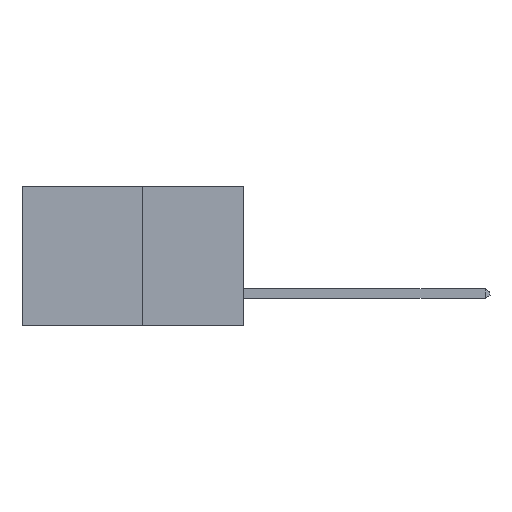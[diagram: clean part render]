
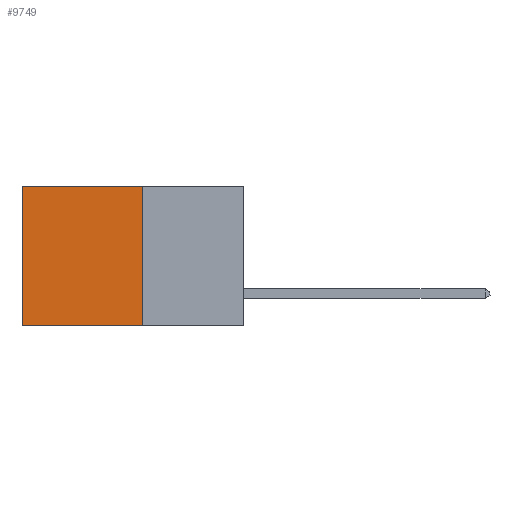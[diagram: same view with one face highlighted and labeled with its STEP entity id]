
A CAD part, left-side view. The second image highlights one B-rep face of the part: STEP entity #9749.
In plain terms, the highlighted planar face has unit normal (-1, 0, 0).
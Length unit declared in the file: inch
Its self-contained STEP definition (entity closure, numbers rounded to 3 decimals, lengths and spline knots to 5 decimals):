
#231 = CARTESIAN_POINT ( 'NONE',  ( 0.277, 0.59, -0.37 ) ) ;
#280 = EDGE_CURVE ( 'NONE', #4749, #3117, #490, .T. ) ;
#294 = ORIENTED_EDGE ( 'NONE', *, *, #6103, .F. ) ;
#366 = AXIS2_PLACEMENT_3D ( 'NONE', #7213, #4935, #9999 ) ;
#490 = LINE ( 'NONE', #6694, #4669 ) ;
#638 = VECTOR ( 'NONE', #7488, 39.37008 ) ;
#659 = EDGE_LOOP ( 'NONE', ( #2244, #294, #944, #1124 ) ) ;
#897 = FACE_OUTER_BOUND ( 'NONE', #659, .T. ) ;
#903 = CARTESIAN_POINT ( 'NONE',  ( 0.277, 0.59, -0.37 ) ) ;
#944 = ORIENTED_EDGE ( 'NONE', *, *, #9655, .F. ) ;
#1052 = VERTEX_POINT ( 'NONE', #7334 ) ;
#1124 = ORIENTED_EDGE ( 'NONE', *, *, #280, .T. ) ;
#1454 = LINE ( 'NONE', #2458, #9580 ) ;
#1643 = LINE ( 'NONE', #5140, #5436 ) ;
#2244 = ORIENTED_EDGE ( 'NONE', *, *, #9331, .T. ) ;
#2458 = CARTESIAN_POINT ( 'NONE',  ( 0.277, 0.27, -0.37 ) ) ;
#2934 = CARTESIAN_POINT ( 'NONE',  ( 0.277, 0.59, 0. ) ) ;
#3117 = VERTEX_POINT ( 'NONE', #2934 ) ;
#4669 = VECTOR ( 'NONE', #6974, 39.37008 ) ;
#4749 = VERTEX_POINT ( 'NONE', #7589 ) ;
#4935 = DIRECTION ( 'NONE',  ( 1., 0., 0. ) ) ;
#5140 = CARTESIAN_POINT ( 'NONE',  ( 0.277, 0.27, -0.37 ) ) ;
#5240 = DIRECTION ( 'NONE',  ( 0., 1., 0. ) ) ;
#5436 = VECTOR ( 'NONE', #5240, 39.37008 ) ;
#5691 = PLANE ( 'NONE',  #366 ) ;
#6103 = EDGE_CURVE ( 'NONE', #1052, #9825, #1643, .T. ) ;
#6694 = CARTESIAN_POINT ( 'NONE',  ( 0.277, 0.27, 0. ) ) ;
#6974 = DIRECTION ( 'NONE',  ( 0., 1., 0. ) ) ;
#7213 = CARTESIAN_POINT ( 'NONE',  ( 0.277, 0.27, -0.37 ) ) ;
#7293 = LINE ( 'NONE', #231, #638 ) ;
#7334 = CARTESIAN_POINT ( 'NONE',  ( 0.277, 0.27, -0.37 ) ) ;
#7488 = DIRECTION ( 'NONE',  ( 0., 0., -1. ) ) ;
#7589 = CARTESIAN_POINT ( 'NONE',  ( 0.277, 0.27, 0. ) ) ;
#7917 = DIRECTION ( 'NONE',  ( 0., 0., -1. ) ) ;
#9331 = EDGE_CURVE ( 'NONE', #3117, #9825, #7293, .T. ) ;
#9580 = VECTOR ( 'NONE', #7917, 39.37008 ) ;
#9655 = EDGE_CURVE ( 'NONE', #4749, #1052, #1454, .T. ) ;
#9749 = ADVANCED_FACE ( 'NONE', ( #897 ), #5691, .F. ) ;
#9825 = VERTEX_POINT ( 'NONE', #903 ) ;
#9999 = DIRECTION ( 'NONE',  ( 0., 0., -1. ) ) ;
